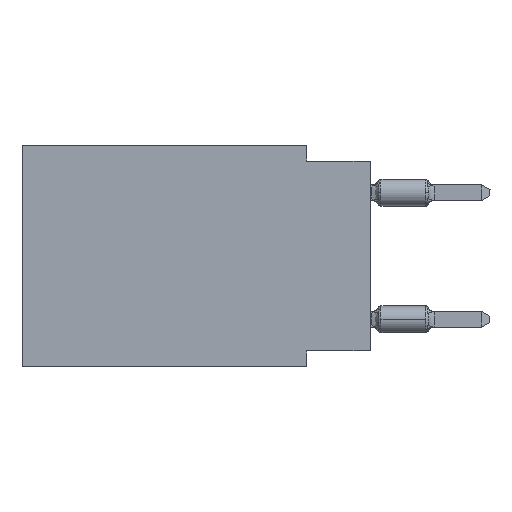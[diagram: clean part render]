
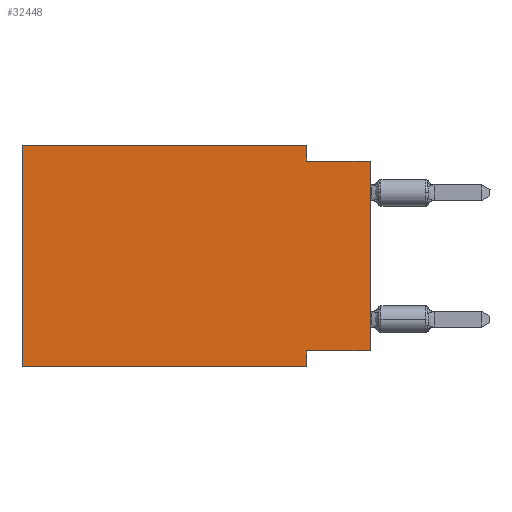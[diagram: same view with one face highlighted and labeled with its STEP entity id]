
A CAD part, left-side view. The second image highlights one B-rep face of the part: STEP entity #32448.
In plain terms, the highlighted planar face has unit normal (-1, 0, 0).
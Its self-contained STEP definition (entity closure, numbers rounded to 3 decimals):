
#1148 = VERTEX_POINT ( 'NONE', #26925 ) ;
#3435 = FACE_OUTER_BOUND ( 'NONE', #34263, .T. ) ;
#4364 = CARTESIAN_POINT ( 'NONE',  ( 0., 0., -0.635 ) ) ;
#4705 = EDGE_CURVE ( 'NONE', #40520, #44764, #43734, .T. ) ;
#5018 = DIRECTION ( 'NONE',  ( 0., -1., 0. ) ) ;
#5193 = CARTESIAN_POINT ( 'NONE',  ( 0., 0., -0.635 ) ) ;
#6749 = CARTESIAN_POINT ( 'NONE',  ( 0., 2.54, 0. ) ) ;
#7326 = VECTOR ( 'NONE', #15030, 1000. ) ;
#7433 = DIRECTION ( 'NONE',  ( 1., 0., 0. ) ) ;
#7482 = EDGE_CURVE ( 'NONE', #25665, #44764, #28752, .T. ) ;
#7731 = CARTESIAN_POINT ( 'NONE',  ( 0., 0., -8.255 ) ) ;
#7801 = EDGE_CURVE ( 'NONE', #30575, #9475, #38653, .T. ) ;
#9475 = VERTEX_POINT ( 'NONE', #16425 ) ;
#11045 = DIRECTION ( 'NONE',  ( 0., 1., 0. ) ) ;
#11405 = ORIENTED_EDGE ( 'NONE', *, *, #26120, .F. ) ;
#12582 = LINE ( 'NONE', #36704, #21570 ) ;
#12864 = EDGE_CURVE ( 'NONE', #27919, #21739, #22583, .T. ) ;
#12884 = ORIENTED_EDGE ( 'NONE', *, *, #4705, .T. ) ;
#15030 = DIRECTION ( 'NONE',  ( 0., 0., -1. ) ) ;
#15125 = ORIENTED_EDGE ( 'NONE', *, *, #7801, .F. ) ;
#15959 = CARTESIAN_POINT ( 'NONE',  ( 0., 0., 0. ) ) ;
#16215 = AXIS2_PLACEMENT_3D ( 'NONE', #28719, #7433, #22082 ) ;
#16425 = CARTESIAN_POINT ( 'NONE',  ( 0., 2.54, -0.635 ) ) ;
#17116 = DIRECTION ( 'NONE',  ( 0., 0., -1. ) ) ;
#18162 = DIRECTION ( 'NONE',  ( 0., -1., 0. ) ) ;
#18467 = ORIENTED_EDGE ( 'NONE', *, *, #20236, .F. ) ;
#19500 = CARTESIAN_POINT ( 'NONE',  ( 0., 13.97, -8.89 ) ) ;
#19851 = DIRECTION ( 'NONE',  ( 0., 0., 1. ) ) ;
#20236 = EDGE_CURVE ( 'NONE', #1148, #30575, #12582, .T. ) ;
#21570 = VECTOR ( 'NONE', #5018, 1000. ) ;
#21739 = VERTEX_POINT ( 'NONE', #4364 ) ;
#22082 = DIRECTION ( 'NONE',  ( 0., 0., -1. ) ) ;
#22583 = LINE ( 'NONE', #15959, #37856 ) ;
#22935 = LINE ( 'NONE', #38075, #38593 ) ;
#23058 = DIRECTION ( 'NONE',  ( 0., 0., 1. ) ) ;
#23169 = EDGE_CURVE ( 'NONE', #27919, #25665, #29252, .T. ) ;
#24480 = ORIENTED_EDGE ( 'NONE', *, *, #12864, .T. ) ;
#25665 = VERTEX_POINT ( 'NONE', #38592 ) ;
#26120 = EDGE_CURVE ( 'NONE', #40520, #1148, #22935, .T. ) ;
#26925 = CARTESIAN_POINT ( 'NONE',  ( 0., 13.97, 0. ) ) ;
#26961 = VECTOR ( 'NONE', #11045, 1000. ) ;
#27919 = VERTEX_POINT ( 'NONE', #45270 ) ;
#28719 = CARTESIAN_POINT ( 'NONE',  ( 0., 13.97, 0. ) ) ;
#28752 = LINE ( 'NONE', #36775, #7326 ) ;
#29252 = LINE ( 'NONE', #7731, #26961 ) ;
#30260 = DIRECTION ( 'NONE',  ( 0., -1., 0. ) ) ;
#30575 = VERTEX_POINT ( 'NONE', #6749 ) ;
#31271 = VECTOR ( 'NONE', #30260, 1000. ) ;
#31988 = ORIENTED_EDGE ( 'NONE', *, *, #23169, .F. ) ;
#32448 = ADVANCED_FACE ( 'NONE', ( #3435 ), #32490, .F. ) ;
#32490 = PLANE ( 'NONE',  #16215 ) ;
#32801 = CARTESIAN_POINT ( 'NONE',  ( 0., 2.54, -8.89 ) ) ;
#32846 = VECTOR ( 'NONE', #18162, 1000. ) ;
#34263 = EDGE_LOOP ( 'NONE', ( #24480, #45441, #15125, #18467, #11405, #12884, #42684, #31988 ) ) ;
#34738 = LINE ( 'NONE', #5193, #31271 ) ;
#36704 = CARTESIAN_POINT ( 'NONE',  ( 0., 13.97, 0. ) ) ;
#36775 = CARTESIAN_POINT ( 'NONE',  ( 0., 2.54, -8.89 ) ) ;
#37856 = VECTOR ( 'NONE', #23058, 1000. ) ;
#38075 = CARTESIAN_POINT ( 'NONE',  ( 0., 13.97, 0. ) ) ;
#38592 = CARTESIAN_POINT ( 'NONE',  ( 0., 2.54, -8.255 ) ) ;
#38593 = VECTOR ( 'NONE', #19851, 1000. ) ;
#38653 = LINE ( 'NONE', #45768, #44355 ) ;
#40173 = CARTESIAN_POINT ( 'NONE',  ( 0., 13.97, -8.89 ) ) ;
#40520 = VERTEX_POINT ( 'NONE', #19500 ) ;
#42684 = ORIENTED_EDGE ( 'NONE', *, *, #7482, .F. ) ;
#43734 = LINE ( 'NONE', #40173, #32846 ) ;
#44355 = VECTOR ( 'NONE', #17116, 1000. ) ;
#44764 = VERTEX_POINT ( 'NONE', #32801 ) ;
#45270 = CARTESIAN_POINT ( 'NONE',  ( 0., 0., -8.255 ) ) ;
#45441 = ORIENTED_EDGE ( 'NONE', *, *, #46681, .F. ) ;
#45768 = CARTESIAN_POINT ( 'NONE',  ( 0., 2.54, 0. ) ) ;
#46681 = EDGE_CURVE ( 'NONE', #9475, #21739, #34738, .T. ) ;
